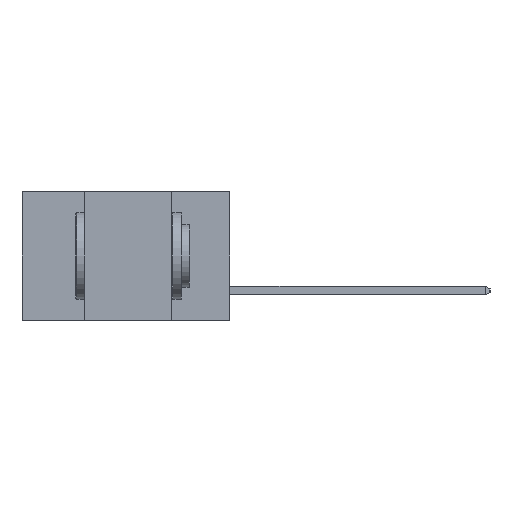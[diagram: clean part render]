
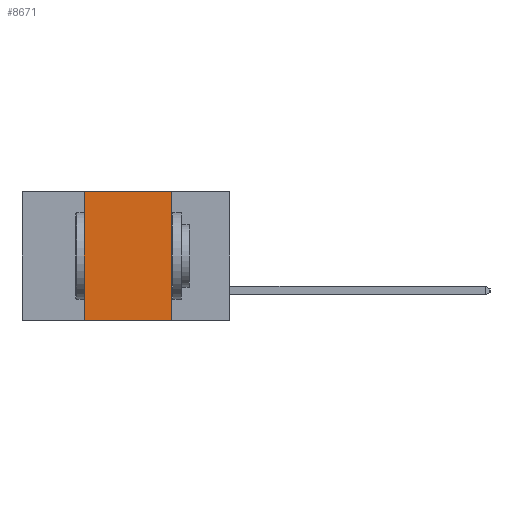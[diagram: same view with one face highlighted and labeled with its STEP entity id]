
A CAD part, left-side view. The second image highlights one B-rep face of the part: STEP entity #8671.
In plain terms, the highlighted planar face has unit normal (-1, 0, 0).
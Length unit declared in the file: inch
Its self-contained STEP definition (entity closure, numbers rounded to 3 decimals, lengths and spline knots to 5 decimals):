
#175 = CARTESIAN_POINT ( 'NONE',  ( 0., 0.17, 0. ) ) ;
#726 = VECTOR ( 'NONE', #2261, 39.37008 ) ;
#1714 = CARTESIAN_POINT ( 'NONE',  ( 0., 0.17, -0.37 ) ) ;
#1928 = PLANE ( 'NONE',  #6554 ) ;
#2261 = DIRECTION ( 'NONE',  ( 0., 0., 1. ) ) ;
#2601 = CARTESIAN_POINT ( 'NONE',  ( 0., 0.42, -0.37 ) ) ;
#3296 = DIRECTION ( 'NONE',  ( 0., 0., -1. ) ) ;
#3514 = LINE ( 'NONE', #6303, #726 ) ;
#3574 = FACE_OUTER_BOUND ( 'NONE', #16074, .T. ) ;
#3733 = VERTEX_POINT ( 'NONE', #1714 ) ;
#4095 = LINE ( 'NONE', #14044, #14128 ) ;
#4147 = VERTEX_POINT ( 'NONE', #175 ) ;
#4790 = EDGE_CURVE ( 'NONE', #9264, #4147, #12877, .T. ) ;
#5128 = EDGE_CURVE ( 'NONE', #11660, #3733, #4095, .T. ) ;
#5394 = ORIENTED_EDGE ( 'NONE', *, *, #4790, .F. ) ;
#5424 = DIRECTION ( 'NONE',  ( 0., 0., -1. ) ) ;
#5859 = DIRECTION ( 'NONE',  ( 0., -1., 0. ) ) ;
#5941 = CARTESIAN_POINT ( 'NONE',  ( 0., 0.6, 0. ) ) ;
#6303 = CARTESIAN_POINT ( 'NONE',  ( 0., 0.42, -0.37 ) ) ;
#6554 = AXIS2_PLACEMENT_3D ( 'NONE', #5941, #11410, #3296 ) ;
#6833 = ORIENTED_EDGE ( 'NONE', *, *, #5128, .T. ) ;
#7519 = EDGE_CURVE ( 'NONE', #4147, #3733, #11237, .T. ) ;
#7546 = ORIENTED_EDGE ( 'NONE', *, *, #7519, .F. ) ;
#7648 = DIRECTION ( 'NONE',  ( 0., -1., 0. ) ) ;
#8101 = CARTESIAN_POINT ( 'NONE',  ( 0., 0.17, -0.37 ) ) ;
#8368 = VECTOR ( 'NONE', #7648, 39.37008 ) ;
#8432 = ORIENTED_EDGE ( 'NONE', *, *, #15193, .F. ) ;
#8671 = ADVANCED_FACE ( 'NONE', ( #3574 ), #1928, .F. ) ;
#9264 = VERTEX_POINT ( 'NONE', #16715 ) ;
#10373 = CARTESIAN_POINT ( 'NONE',  ( 0., 0.6, 0. ) ) ;
#11237 = LINE ( 'NONE', #8101, #11675 ) ;
#11410 = DIRECTION ( 'NONE',  ( 1., 0., 0. ) ) ;
#11660 = VERTEX_POINT ( 'NONE', #2601 ) ;
#11675 = VECTOR ( 'NONE', #5424, 39.37008 ) ;
#12877 = LINE ( 'NONE', #10373, #8368 ) ;
#14044 = CARTESIAN_POINT ( 'NONE',  ( 0., 0.6, -0.37 ) ) ;
#14128 = VECTOR ( 'NONE', #5859, 39.37008 ) ;
#15193 = EDGE_CURVE ( 'NONE', #11660, #9264, #3514, .T. ) ;
#16074 = EDGE_LOOP ( 'NONE', ( #7546, #5394, #8432, #6833 ) ) ;
#16715 = CARTESIAN_POINT ( 'NONE',  ( 0., 0.42, 0. ) ) ;
